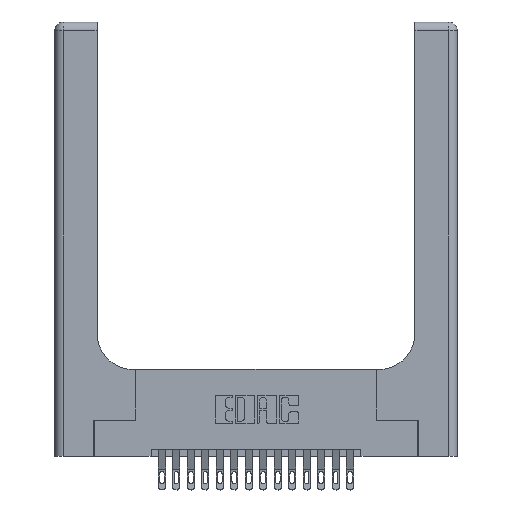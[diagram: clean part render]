
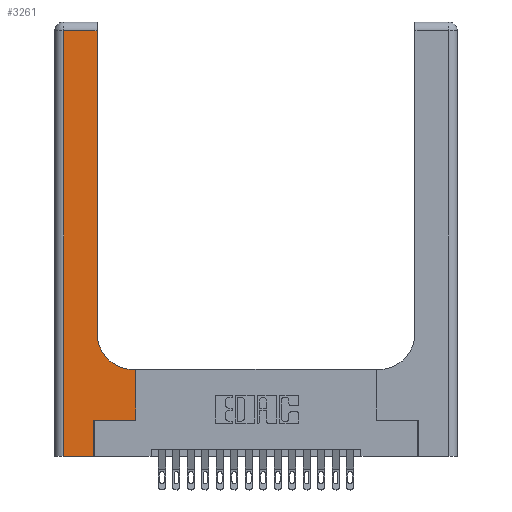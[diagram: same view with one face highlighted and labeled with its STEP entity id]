
A CAD part, top view. The second image highlights one B-rep face of the part: STEP entity #3261.
In plain terms, the highlighted planar face has unit normal (0, 0, 1).
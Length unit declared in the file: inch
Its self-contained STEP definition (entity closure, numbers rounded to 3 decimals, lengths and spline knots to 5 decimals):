
#141 = CARTESIAN_POINT ( 'NONE',  ( 0.269, 0.25, 0.37 ) ) ;
#245 = DIRECTION ( 'NONE',  ( 0., 0., -1. ) ) ;
#308 = CARTESIAN_POINT ( 'NONE',  ( 0.269, 0.25, 0.37 ) ) ;
#362 = CARTESIAN_POINT ( 'NONE',  ( 0.2915, 3., 0.37 ) ) ;
#1378 = LINE ( 'NONE', #7937, #9393 ) ;
#1735 = DIRECTION ( 'NONE',  ( 0., 1., 0. ) ) ;
#2031 = VERTEX_POINT ( 'NONE', #141 ) ;
#2264 = ORIENTED_EDGE ( 'NONE', *, *, #13837, .T. ) ;
#2377 = LINE ( 'NONE', #11124, #14862 ) ;
#2458 = VERTEX_POINT ( 'NONE', #13824 ) ;
#2935 = ORIENTED_EDGE ( 'NONE', *, *, #7357, .T. ) ;
#2945 = DIRECTION ( 'NONE',  ( -1., 0., 0. ) ) ;
#2991 = FACE_OUTER_BOUND ( 'NONE', #14328, .T. ) ;
#3252 = EDGE_CURVE ( 'NONE', #17829, #17123, #16936, .T. ) ;
#3261 = ADVANCED_FACE ( 'NONE', ( #2991 ), #3274, .F. ) ;
#3274 = PLANE ( 'NONE',  #13841 ) ;
#3420 = DIRECTION ( 'NONE',  ( 0., 1., 0. ) ) ;
#4133 = CIRCLE ( 'NONE', #19369, 0.25 ) ;
#4137 = ORIENTED_EDGE ( 'NONE', *, *, #9055, .T. ) ;
#4833 = CARTESIAN_POINT ( 'NONE',  ( 0., 3., 0.37 ) ) ;
#4863 = ORIENTED_EDGE ( 'NONE', *, *, #3252, .T. ) ;
#4988 = VECTOR ( 'NONE', #8334, 39.37008 ) ;
#5036 = LINE ( 'NONE', #12284, #12867 ) ;
#5049 = EDGE_CURVE ( 'NONE', #17331, #20029, #5036, .T. ) ;
#5355 = ORIENTED_EDGE ( 'NONE', *, *, #11538, .T. ) ;
#7357 = EDGE_CURVE ( 'NONE', #20029, #2458, #17450, .T. ) ;
#7820 = DIRECTION ( 'NONE',  ( -1., 0., 0. ) ) ;
#7870 = CARTESIAN_POINT ( 'NONE',  ( 0.2915, 2.94, 0.37 ) ) ;
#7937 = CARTESIAN_POINT ( 'NONE',  ( 0.5585, 0.25, 0.37 ) ) ;
#8224 = CARTESIAN_POINT ( 'NONE',  ( 0.5585, 0.25, 0.37 ) ) ;
#8334 = DIRECTION ( 'NONE',  ( 0., -1., 0. ) ) ;
#9055 = EDGE_CURVE ( 'NONE', #2458, #18072, #11492, .T. ) ;
#9393 = VECTOR ( 'NONE', #1735, 39.37008 ) ;
#10529 = EDGE_CURVE ( 'NONE', #17123, #13040, #4133, .T. ) ;
#10768 = VECTOR ( 'NONE', #11344, 39.37008 ) ;
#11033 = CARTESIAN_POINT ( 'NONE',  ( 0.2915, 0.6, 0.37 ) ) ;
#11056 = CARTESIAN_POINT ( 'NONE',  ( 0.5415, 0.85, 0.37 ) ) ;
#11124 = CARTESIAN_POINT ( 'NONE',  ( 0.269, 0., 0.37 ) ) ;
#11344 = DIRECTION ( 'NONE',  ( 0., 1., 0. ) ) ;
#11492 = LINE ( 'NONE', #12660, #14207 ) ;
#11538 = EDGE_CURVE ( 'NONE', #18072, #2031, #2377, .T. ) ;
#11667 = CARTESIAN_POINT ( 'NONE',  ( 0.269, 0., 0.37 ) ) ;
#12248 = ORIENTED_EDGE ( 'NONE', *, *, #10529, .T. ) ;
#12284 = CARTESIAN_POINT ( 'NONE',  ( 0., 2.94, 0.37 ) ) ;
#12660 = CARTESIAN_POINT ( 'NONE',  ( 0., 0., 0.37 ) ) ;
#12724 = EDGE_CURVE ( 'NONE', #18539, #17829, #1378, .T. ) ;
#12764 = VECTOR ( 'NONE', #7820, 39.37008 ) ;
#12867 = VECTOR ( 'NONE', #2945, 39.37008 ) ;
#13040 = VERTEX_POINT ( 'NONE', #16846 ) ;
#13120 = CARTESIAN_POINT ( 'NONE',  ( 0.06, 2.94, 0.37 ) ) ;
#13343 = ORIENTED_EDGE ( 'NONE', *, *, #12724, .T. ) ;
#13406 = ORIENTED_EDGE ( 'NONE', *, *, #5049, .T. ) ;
#13824 = CARTESIAN_POINT ( 'NONE',  ( 0.06, 0., 0.37 ) ) ;
#13837 = EDGE_CURVE ( 'NONE', #2031, #18539, #14765, .T. ) ;
#13841 = AXIS2_PLACEMENT_3D ( 'NONE', #4833, #245, #15791 ) ;
#14207 = VECTOR ( 'NONE', #15684, 39.37008 ) ;
#14328 = EDGE_LOOP ( 'NONE', ( #15186, #13406, #2935, #4137, #5355, #2264, #13343, #4863, #12248 ) ) ;
#14524 = VECTOR ( 'NONE', #15923, 39.37008 ) ;
#14765 = LINE ( 'NONE', #308, #14524 ) ;
#14862 = VECTOR ( 'NONE', #3420, 39.37008 ) ;
#15098 = CARTESIAN_POINT ( 'NONE',  ( 0.5415, 0.6, 0.37 ) ) ;
#15186 = ORIENTED_EDGE ( 'NONE', *, *, #17504, .T. ) ;
#15212 = LINE ( 'NONE', #362, #10768 ) ;
#15346 = CARTESIAN_POINT ( 'NONE',  ( 0.5585, 0.6, 0.37 ) ) ;
#15684 = DIRECTION ( 'NONE',  ( 1., 0., 0. ) ) ;
#15791 = DIRECTION ( 'NONE',  ( -1., 0., 0. ) ) ;
#15883 = DIRECTION ( 'NONE',  ( 0., 0., -1. ) ) ;
#15923 = DIRECTION ( 'NONE',  ( 1., 0., 0. ) ) ;
#16313 = CARTESIAN_POINT ( 'NONE',  ( 0.06, 3., 0.37 ) ) ;
#16846 = CARTESIAN_POINT ( 'NONE',  ( 0.2915, 0.85, 0.37 ) ) ;
#16936 = LINE ( 'NONE', #11033, #12764 ) ;
#17123 = VERTEX_POINT ( 'NONE', #15098 ) ;
#17164 = DIRECTION ( 'NONE',  ( 1., 0., 0. ) ) ;
#17331 = VERTEX_POINT ( 'NONE', #7870 ) ;
#17450 = LINE ( 'NONE', #16313, #4988 ) ;
#17504 = EDGE_CURVE ( 'NONE', #13040, #17331, #15212, .T. ) ;
#17829 = VERTEX_POINT ( 'NONE', #15346 ) ;
#18072 = VERTEX_POINT ( 'NONE', #11667 ) ;
#18539 = VERTEX_POINT ( 'NONE', #8224 ) ;
#19369 = AXIS2_PLACEMENT_3D ( 'NONE', #11056, #15883, #17164 ) ;
#20029 = VERTEX_POINT ( 'NONE', #13120 ) ;
